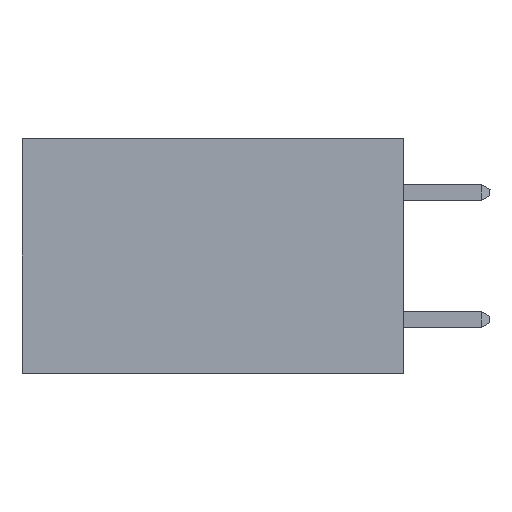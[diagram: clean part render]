
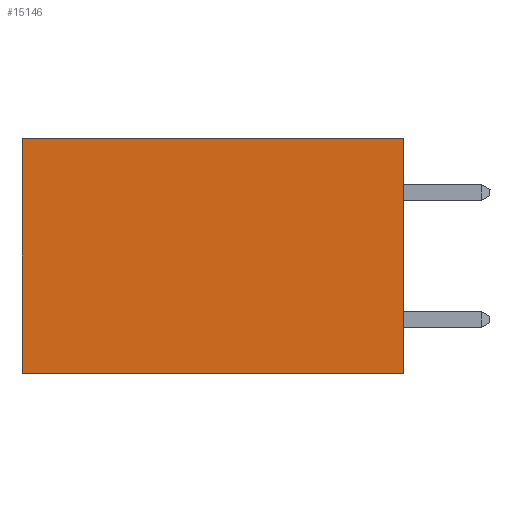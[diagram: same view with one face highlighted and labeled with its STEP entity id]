
A CAD part, left-side view. The second image highlights one B-rep face of the part: STEP entity #15146.
In plain terms, the highlighted planar face has unit normal (-1, 0, 0).
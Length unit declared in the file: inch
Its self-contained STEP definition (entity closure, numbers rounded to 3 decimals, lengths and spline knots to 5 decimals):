
#410 = EDGE_CURVE ( 'NONE', #5322, #4532, #570, .T. ) ;
#570 = LINE ( 'NONE', #5779, #11580 ) ;
#2158 = PLANE ( 'NONE',  #5344 ) ;
#2726 = FACE_OUTER_BOUND ( 'NONE', #6077, .T. ) ;
#2938 = ORIENTED_EDGE ( 'NONE', *, *, #410, .T. ) ;
#4492 = VECTOR ( 'NONE', #10155, 39.37008 ) ;
#4532 = VERTEX_POINT ( 'NONE', #9362 ) ;
#5115 = CARTESIAN_POINT ( 'NONE',  ( 0.2875, 0., -0.37 ) ) ;
#5133 = DIRECTION ( 'NONE',  ( 1., 0., 0. ) ) ;
#5322 = VERTEX_POINT ( 'NONE', #16808 ) ;
#5344 = AXIS2_PLACEMENT_3D ( 'NONE', #13646, #5133, #15073 ) ;
#5541 = DIRECTION ( 'NONE',  ( 0., 0., -1. ) ) ;
#5779 = CARTESIAN_POINT ( 'NONE',  ( 0.2875, 0.6, 0. ) ) ;
#6077 = EDGE_LOOP ( 'NONE', ( #2938, #14955, #17327, #8602 ) ) ;
#6919 = EDGE_CURVE ( 'NONE', #7020, #5322, #17401, .T. ) ;
#7020 = VERTEX_POINT ( 'NONE', #14699 ) ;
#8241 = LINE ( 'NONE', #8716, #4492 ) ;
#8602 = ORIENTED_EDGE ( 'NONE', *, *, #6919, .T. ) ;
#8716 = CARTESIAN_POINT ( 'NONE',  ( 0.2875, 0., 0. ) ) ;
#9362 = CARTESIAN_POINT ( 'NONE',  ( 0.2875, 0.6, -0.37 ) ) ;
#9881 = VECTOR ( 'NONE', #11712, 39.37008 ) ;
#9955 = CARTESIAN_POINT ( 'NONE',  ( 0.2875, 0., -0.37 ) ) ;
#10155 = DIRECTION ( 'NONE',  ( 0., 0., -1. ) ) ;
#10273 = CARTESIAN_POINT ( 'NONE',  ( 0.2875, 0., 0. ) ) ;
#11059 = EDGE_CURVE ( 'NONE', #7020, #18280, #8241, .T. ) ;
#11580 = VECTOR ( 'NONE', #5541, 39.37008 ) ;
#11712 = DIRECTION ( 'NONE',  ( 0., 1., 0. ) ) ;
#12068 = VECTOR ( 'NONE', #16496, 39.37008 ) ;
#12532 = LINE ( 'NONE', #5115, #12068 ) ;
#13646 = CARTESIAN_POINT ( 'NONE',  ( 0.2875, 0., 0. ) ) ;
#14699 = CARTESIAN_POINT ( 'NONE',  ( 0.2875, 0., 0. ) ) ;
#14955 = ORIENTED_EDGE ( 'NONE', *, *, #16793, .F. ) ;
#15073 = DIRECTION ( 'NONE',  ( 0., 0., -1. ) ) ;
#15146 = ADVANCED_FACE ( 'NONE', ( #2726 ), #2158, .F. ) ;
#16496 = DIRECTION ( 'NONE',  ( 0., 1., 0. ) ) ;
#16793 = EDGE_CURVE ( 'NONE', #18280, #4532, #12532, .T. ) ;
#16808 = CARTESIAN_POINT ( 'NONE',  ( 0.2875, 0.6, 0. ) ) ;
#17327 = ORIENTED_EDGE ( 'NONE', *, *, #11059, .F. ) ;
#17401 = LINE ( 'NONE', #10273, #9881 ) ;
#18280 = VERTEX_POINT ( 'NONE', #9955 ) ;
